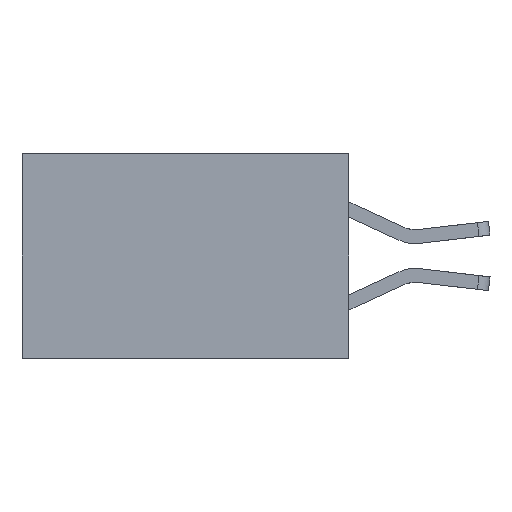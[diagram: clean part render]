
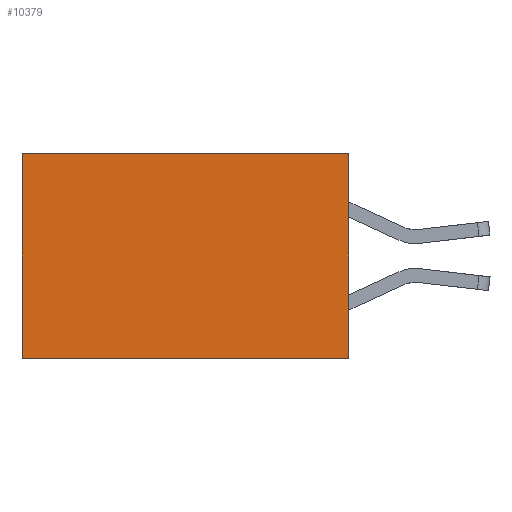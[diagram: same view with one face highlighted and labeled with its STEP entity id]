
A CAD part, left-side view. The second image highlights one B-rep face of the part: STEP entity #10379.
In plain terms, the highlighted planar face has unit normal (-1, 0, 0).
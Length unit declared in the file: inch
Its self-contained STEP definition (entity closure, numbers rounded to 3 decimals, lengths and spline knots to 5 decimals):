
#5 = EDGE_CURVE ( 'NONE', #5001, #9073, #9240, .T. ) ;
#523 = EDGE_CURVE ( 'NONE', #9225, #5001, #8884, .T. ) ;
#1657 = ORIENTED_EDGE ( 'NONE', *, *, #5, .T. ) ;
#1863 = EDGE_CURVE ( 'NONE', #9225, #12910, #5072, .T. ) ;
#2921 = CARTESIAN_POINT ( 'NONE',  ( 0.277, 0., -0.37 ) ) ;
#3295 = VECTOR ( 'NONE', #13582, 39.37008 ) ;
#4148 = CARTESIAN_POINT ( 'NONE',  ( 0.277, 0.59, 0. ) ) ;
#4960 = ORIENTED_EDGE ( 'NONE', *, *, #523, .T. ) ;
#5001 = VERTEX_POINT ( 'NONE', #4148 ) ;
#5072 = LINE ( 'NONE', #9616, #8220 ) ;
#5178 = FACE_OUTER_BOUND ( 'NONE', #12831, .T. ) ;
#5345 = VECTOR ( 'NONE', #8366, 39.37008 ) ;
#5423 = ORIENTED_EDGE ( 'NONE', *, *, #1863, .F. ) ;
#6211 = CARTESIAN_POINT ( 'NONE',  ( 0.277, 0., 0. ) ) ;
#6219 = CARTESIAN_POINT ( 'NONE',  ( 0.277, 0., -0.37 ) ) ;
#6395 = VECTOR ( 'NONE', #7590, 39.37008 ) ;
#6451 = AXIS2_PLACEMENT_3D ( 'NONE', #11880, #12891, #6623 ) ;
#6577 = PLANE ( 'NONE',  #6451 ) ;
#6623 = DIRECTION ( 'NONE',  ( 0., 0., -1. ) ) ;
#7590 = DIRECTION ( 'NONE',  ( 0., 0., -1. ) ) ;
#8150 = DIRECTION ( 'NONE',  ( 0., 0., -1. ) ) ;
#8170 = LINE ( 'NONE', #6219, #5345 ) ;
#8220 = VECTOR ( 'NONE', #8150, 39.37008 ) ;
#8366 = DIRECTION ( 'NONE',  ( 0., 1., 0. ) ) ;
#8840 = CARTESIAN_POINT ( 'NONE',  ( 0.277, 0., 0. ) ) ;
#8884 = LINE ( 'NONE', #6211, #3295 ) ;
#9073 = VERTEX_POINT ( 'NONE', #11768 ) ;
#9225 = VERTEX_POINT ( 'NONE', #8840 ) ;
#9240 = LINE ( 'NONE', #9698, #6395 ) ;
#9616 = CARTESIAN_POINT ( 'NONE',  ( 0.277, 0., -0.37 ) ) ;
#9698 = CARTESIAN_POINT ( 'NONE',  ( 0.277, 0.59, -0.37 ) ) ;
#10101 = EDGE_CURVE ( 'NONE', #12910, #9073, #8170, .T. ) ;
#10379 = ADVANCED_FACE ( 'NONE', ( #5178 ), #6577, .F. ) ;
#11768 = CARTESIAN_POINT ( 'NONE',  ( 0.277, 0.59, -0.37 ) ) ;
#11880 = CARTESIAN_POINT ( 'NONE',  ( 0.277, 0., -0.37 ) ) ;
#12804 = ORIENTED_EDGE ( 'NONE', *, *, #10101, .F. ) ;
#12831 = EDGE_LOOP ( 'NONE', ( #1657, #12804, #5423, #4960 ) ) ;
#12891 = DIRECTION ( 'NONE',  ( 1., 0., 0. ) ) ;
#12910 = VERTEX_POINT ( 'NONE', #2921 ) ;
#13582 = DIRECTION ( 'NONE',  ( 0., 1., 0. ) ) ;
